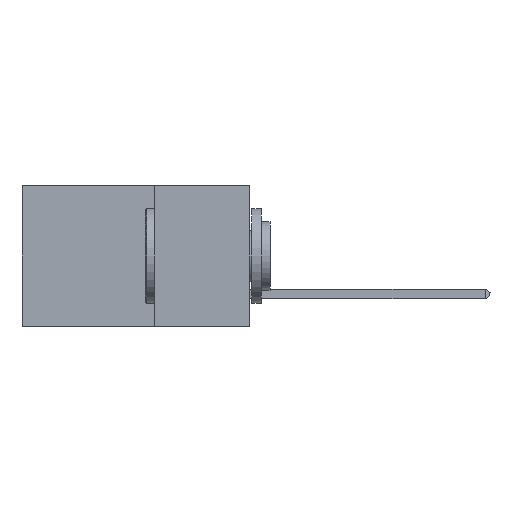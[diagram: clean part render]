
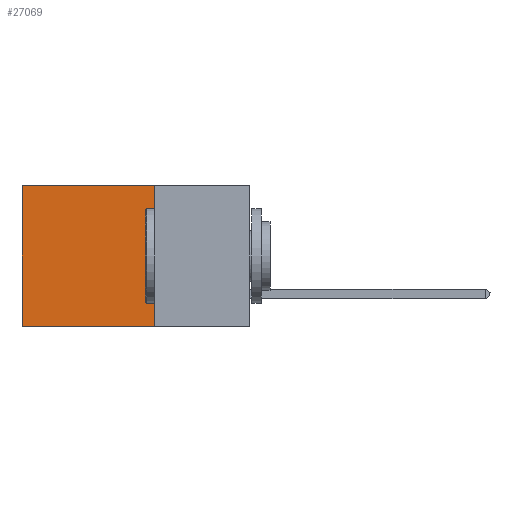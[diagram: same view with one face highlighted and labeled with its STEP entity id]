
A CAD part, left-side view. The second image highlights one B-rep face of the part: STEP entity #27069.
In plain terms, the highlighted planar face has unit normal (-1, 0, 0).
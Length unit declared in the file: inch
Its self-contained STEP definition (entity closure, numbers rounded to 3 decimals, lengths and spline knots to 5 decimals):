
#32 = VECTOR ( 'NONE', #37377, 39.37008 ) ;
#973 = LINE ( 'NONE', #14395, #32459 ) ;
#982 = CARTESIAN_POINT ( 'NONE',  ( 0.2875, 0.6, 0. ) ) ;
#2712 = VERTEX_POINT ( 'NONE', #17716 ) ;
#4698 = DIRECTION ( 'NONE',  ( 0., 1., 0. ) ) ;
#5206 = LINE ( 'NONE', #24909, #29891 ) ;
#8008 = ORIENTED_EDGE ( 'NONE', *, *, #42400, .F. ) ;
#9581 = CARTESIAN_POINT ( 'NONE',  ( 0.2875, 0.6, -0.37 ) ) ;
#9797 = FACE_OUTER_BOUND ( 'NONE', #13636, .T. ) ;
#9812 = LINE ( 'NONE', #33864, #32 ) ;
#11707 = EDGE_CURVE ( 'NONE', #2712, #38208, #5206, .T. ) ;
#11836 = CARTESIAN_POINT ( 'NONE',  ( 0.2875, 0.25, -0.37 ) ) ;
#13626 = CARTESIAN_POINT ( 'NONE',  ( 0.2875, 0.25, 0. ) ) ;
#13636 = EDGE_LOOP ( 'NONE', ( #37039, #25837, #8008, #39876 ) ) ;
#14395 = CARTESIAN_POINT ( 'NONE',  ( 0.2875, 0.25, -0.37 ) ) ;
#14745 = DIRECTION ( 'NONE',  ( 0., 1., 0. ) ) ;
#15432 = EDGE_CURVE ( 'NONE', #38208, #24359, #20557, .T. ) ;
#16990 = VECTOR ( 'NONE', #21686, 39.37008 ) ;
#17716 = CARTESIAN_POINT ( 'NONE',  ( 0.2875, 0.25, 0. ) ) ;
#18639 = CARTESIAN_POINT ( 'NONE',  ( 0.2875, 0.6, 0. ) ) ;
#20557 = LINE ( 'NONE', #18639, #16990 ) ;
#21686 = DIRECTION ( 'NONE',  ( 0., 0., -1. ) ) ;
#21849 = VERTEX_POINT ( 'NONE', #11836 ) ;
#24359 = VERTEX_POINT ( 'NONE', #9581 ) ;
#24909 = CARTESIAN_POINT ( 'NONE',  ( 0.2875, 0.25, 0. ) ) ;
#25837 = ORIENTED_EDGE ( 'NONE', *, *, #29782, .F. ) ;
#27069 = ADVANCED_FACE ( 'NONE', ( #9797 ), #33325, .F. ) ;
#29729 = DIRECTION ( 'NONE',  ( 0., 0., -1. ) ) ;
#29782 = EDGE_CURVE ( 'NONE', #21849, #24359, #973, .T. ) ;
#29891 = VECTOR ( 'NONE', #14745, 39.37008 ) ;
#32459 = VECTOR ( 'NONE', #4698, 39.37008 ) ;
#33325 = PLANE ( 'NONE',  #41388 ) ;
#33864 = CARTESIAN_POINT ( 'NONE',  ( 0.2875, 0.25, 0. ) ) ;
#36802 = DIRECTION ( 'NONE',  ( 1., 0., 0. ) ) ;
#37039 = ORIENTED_EDGE ( 'NONE', *, *, #15432, .T. ) ;
#37377 = DIRECTION ( 'NONE',  ( 0., 0., -1. ) ) ;
#38208 = VERTEX_POINT ( 'NONE', #982 ) ;
#39876 = ORIENTED_EDGE ( 'NONE', *, *, #11707, .T. ) ;
#41388 = AXIS2_PLACEMENT_3D ( 'NONE', #13626, #36802, #29729 ) ;
#42400 = EDGE_CURVE ( 'NONE', #2712, #21849, #9812, .T. ) ;
